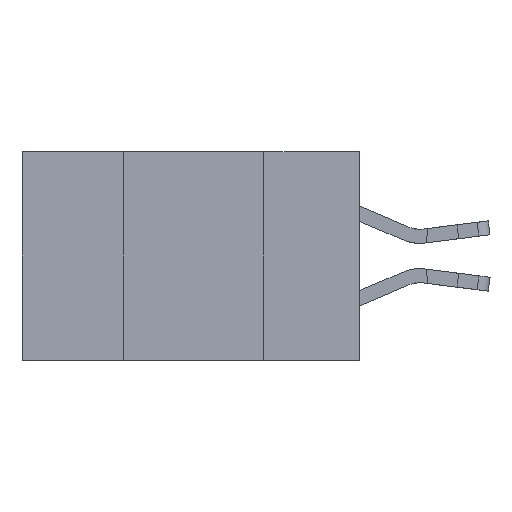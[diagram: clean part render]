
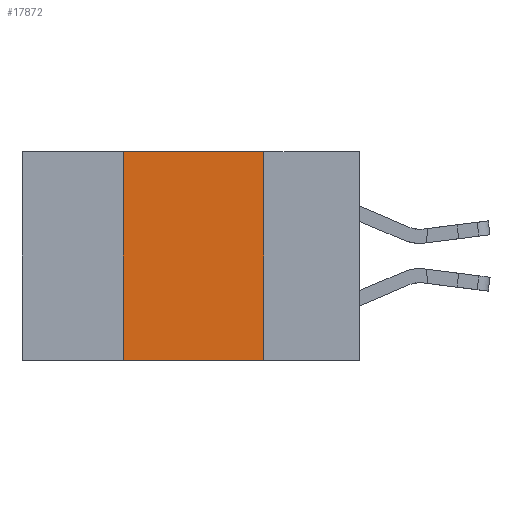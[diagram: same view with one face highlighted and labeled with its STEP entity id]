
A CAD part, left-side view. The second image highlights one B-rep face of the part: STEP entity #17872.
In plain terms, the highlighted planar face has unit normal (-1, 0, 0).
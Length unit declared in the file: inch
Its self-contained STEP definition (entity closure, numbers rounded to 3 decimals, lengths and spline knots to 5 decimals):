
#86 = VECTOR ( 'NONE', #5572, 39.37008 ) ;
#380 = FACE_OUTER_BOUND ( 'NONE', #29643, .T. ) ;
#579 = PLANE ( 'NONE',  #19932 ) ;
#595 = CARTESIAN_POINT ( 'NONE',  ( 0., 0.6, -0.37 ) ) ;
#1052 = DIRECTION ( 'NONE',  ( 0., 0., 1. ) ) ;
#1945 = VERTEX_POINT ( 'NONE', #18233 ) ;
#2752 = ORIENTED_EDGE ( 'NONE', *, *, #26843, .F. ) ;
#3310 = DIRECTION ( 'NONE',  ( 0., 0., -1. ) ) ;
#3855 = EDGE_CURVE ( 'NONE', #1945, #14527, #21772, .T. ) ;
#3868 = CARTESIAN_POINT ( 'NONE',  ( 0., 0.17, -0.37 ) ) ;
#5572 = DIRECTION ( 'NONE',  ( 0., -1., 0. ) ) ;
#6736 = ORIENTED_EDGE ( 'NONE', *, *, #11586, .F. ) ;
#7644 = VECTOR ( 'NONE', #25875, 39.37008 ) ;
#10185 = CARTESIAN_POINT ( 'NONE',  ( 0., 0.6, 0. ) ) ;
#11415 = ORIENTED_EDGE ( 'NONE', *, *, #3855, .F. ) ;
#11586 = EDGE_CURVE ( 'NONE', #24382, #20918, #23985, .T. ) ;
#12702 = CARTESIAN_POINT ( 'NONE',  ( 0., 0.42, 0. ) ) ;
#13258 = LINE ( 'NONE', #10185, #86 ) ;
#14527 = VERTEX_POINT ( 'NONE', #3868 ) ;
#14942 = LINE ( 'NONE', #595, #7644 ) ;
#15256 = VECTOR ( 'NONE', #1052, 39.37008 ) ;
#15449 = CARTESIAN_POINT ( 'NONE',  ( 0., 0.42, 0. ) ) ;
#15538 = DIRECTION ( 'NONE',  ( 0., 0., -1. ) ) ;
#17295 = CARTESIAN_POINT ( 'NONE',  ( 0., 0.6, 0. ) ) ;
#17872 = ADVANCED_FACE ( 'NONE', ( #380 ), #579, .F. ) ;
#18233 = CARTESIAN_POINT ( 'NONE',  ( 0., 0.17, 0. ) ) ;
#19932 = AXIS2_PLACEMENT_3D ( 'NONE', #17295, #28895, #3310 ) ;
#20918 = VERTEX_POINT ( 'NONE', #15449 ) ;
#21772 = LINE ( 'NONE', #22550, #23229 ) ;
#22550 = CARTESIAN_POINT ( 'NONE',  ( 0., 0.17, 0. ) ) ;
#23229 = VECTOR ( 'NONE', #15538, 39.37008 ) ;
#23985 = LINE ( 'NONE', #12702, #15256 ) ;
#24382 = VERTEX_POINT ( 'NONE', #25946 ) ;
#25875 = DIRECTION ( 'NONE',  ( 0., -1., 0. ) ) ;
#25946 = CARTESIAN_POINT ( 'NONE',  ( 0., 0.42, -0.37 ) ) ;
#26295 = ORIENTED_EDGE ( 'NONE', *, *, #28759, .T. ) ;
#26843 = EDGE_CURVE ( 'NONE', #20918, #1945, #13258, .T. ) ;
#28759 = EDGE_CURVE ( 'NONE', #24382, #14527, #14942, .T. ) ;
#28895 = DIRECTION ( 'NONE',  ( 1., 0., 0. ) ) ;
#29643 = EDGE_LOOP ( 'NONE', ( #11415, #2752, #6736, #26295 ) ) ;
